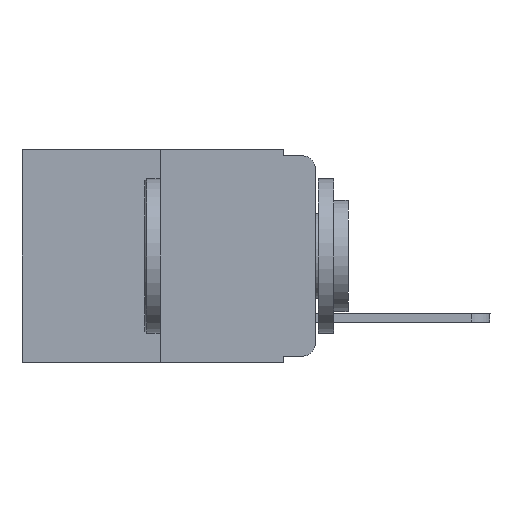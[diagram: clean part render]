
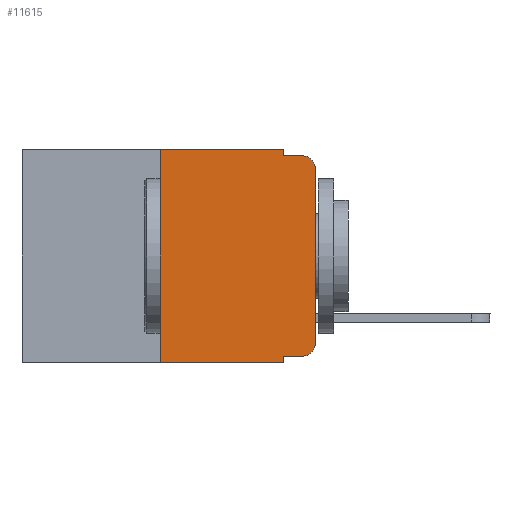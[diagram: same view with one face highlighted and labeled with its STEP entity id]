
A CAD part, left-side view. The second image highlights one B-rep face of the part: STEP entity #11615.
In plain terms, the highlighted planar face has unit normal (-1, 0, 0).
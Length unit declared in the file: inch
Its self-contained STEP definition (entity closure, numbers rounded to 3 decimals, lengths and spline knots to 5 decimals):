
#51 = DIRECTION ( 'NONE',  ( 0., 0., -1. ) ) ;
#181 = CARTESIAN_POINT ( 'NONE',  ( 0., 0.25, 0. ) ) ;
#511 = ORIENTED_EDGE ( 'NONE', *, *, #19440, .T. ) ;
#633 = VECTOR ( 'NONE', #51, 39.37008 ) ;
#698 = VERTEX_POINT ( 'NONE', #17867 ) ;
#1105 = VECTOR ( 'NONE', #6420, 39.37008 ) ;
#1131 = DIRECTION ( 'NONE',  ( 0., 0., -1. ) ) ;
#1224 = VERTEX_POINT ( 'NONE', #16883 ) ;
#1308 = VERTEX_POINT ( 'NONE', #9036 ) ;
#1438 = ORIENTED_EDGE ( 'NONE', *, *, #10637, .F. ) ;
#1750 = DIRECTION ( 'NONE',  ( 0., 0., 1. ) ) ;
#1753 = CARTESIAN_POINT ( 'NONE',  ( 0., 0., 0. ) ) ;
#1965 = EDGE_CURVE ( 'NONE', #13416, #4451, #17871, .T. ) ;
#2322 = CARTESIAN_POINT ( 'NONE',  ( 0., 0.473, -0.343 ) ) ;
#3018 = EDGE_CURVE ( 'NONE', #4451, #4142, #10942, .T. ) ;
#3099 = CARTESIAN_POINT ( 'NONE',  ( 0., 0., -0.313 ) ) ;
#4028 = VERTEX_POINT ( 'NONE', #3099 ) ;
#4041 = CARTESIAN_POINT ( 'NONE',  ( 0., 0.051, -0.01 ) ) ;
#4138 = LINE ( 'NONE', #4041, #8868 ) ;
#4142 = VERTEX_POINT ( 'NONE', #10747 ) ;
#4255 = VECTOR ( 'NONE', #10117, 39.37008 ) ;
#4418 = LINE ( 'NONE', #1753, #1105 ) ;
#4450 = EDGE_CURVE ( 'NONE', #16746, #13416, #20110, .T. ) ;
#4451 = VERTEX_POINT ( 'NONE', #11332 ) ;
#4659 = CARTESIAN_POINT ( 'NONE',  ( 0., 0.051, 0. ) ) ;
#5039 = DIRECTION ( 'NONE',  ( 0., 0., -1. ) ) ;
#5321 = VECTOR ( 'NONE', #13390, 39.37008 ) ;
#5328 = ORIENTED_EDGE ( 'NONE', *, *, #3018, .F. ) ;
#5369 = DIRECTION ( 'NONE',  ( -1., 0., 0. ) ) ;
#5661 = ORIENTED_EDGE ( 'NONE', *, *, #4450, .F. ) ;
#5668 = VECTOR ( 'NONE', #8536, 39.37008 ) ;
#5938 = CIRCLE ( 'NONE', #19613, 0.02 ) ;
#5996 = CARTESIAN_POINT ( 'NONE',  ( 0., 0.25, -0.343 ) ) ;
#6420 = DIRECTION ( 'NONE',  ( 0., 0., 1. ) ) ;
#6889 = EDGE_CURVE ( 'NONE', #12140, #4028, #10310, .T. ) ;
#8536 = DIRECTION ( 'NONE',  ( 0., -1., 0. ) ) ;
#8677 = PLANE ( 'NONE',  #17695 ) ;
#8794 = ORIENTED_EDGE ( 'NONE', *, *, #6889, .T. ) ;
#8868 = VECTOR ( 'NONE', #10045, 39.37008 ) ;
#9036 = CARTESIAN_POINT ( 'NONE',  ( 0., 0.051, -0.343 ) ) ;
#9367 = ORIENTED_EDGE ( 'NONE', *, *, #1965, .F. ) ;
#9650 = EDGE_CURVE ( 'NONE', #1224, #698, #5938, .T. ) ;
#9795 = ORIENTED_EDGE ( 'NONE', *, *, #11631, .T. ) ;
#10045 = DIRECTION ( 'NONE',  ( 0., -1., 0. ) ) ;
#10117 = DIRECTION ( 'NONE',  ( 0., -1., 0. ) ) ;
#10310 = CIRCLE ( 'NONE', #14862, 0.02 ) ;
#10389 = ORIENTED_EDGE ( 'NONE', *, *, #20012, .T. ) ;
#10637 = EDGE_CURVE ( 'NONE', #4142, #698, #4138, .T. ) ;
#10747 = CARTESIAN_POINT ( 'NONE',  ( 0., 0.051, -0.01 ) ) ;
#10942 = LINE ( 'NONE', #14113, #16227 ) ;
#11332 = CARTESIAN_POINT ( 'NONE',  ( 0., 0.051, 0. ) ) ;
#11613 = LINE ( 'NONE', #2322, #5668 ) ;
#11615 = ADVANCED_FACE ( 'NONE', ( #18163 ), #8677, .F. ) ;
#11631 = EDGE_CURVE ( 'NONE', #19550, #12140, #19896, .T. ) ;
#12140 = VERTEX_POINT ( 'NONE', #12539 ) ;
#12160 = CARTESIAN_POINT ( 'NONE',  ( 0., 0.473, 0. ) ) ;
#12397 = DIRECTION ( 'NONE',  ( -1., 0., 0. ) ) ;
#12499 = DIRECTION ( 'NONE',  ( 0., 0., -1. ) ) ;
#12539 = CARTESIAN_POINT ( 'NONE',  ( 0., 0.02, -0.333 ) ) ;
#13133 = DIRECTION ( 'NONE',  ( 0., 0., -1. ) ) ;
#13390 = DIRECTION ( 'NONE',  ( 0., -1., 0. ) ) ;
#13416 = VERTEX_POINT ( 'NONE', #181 ) ;
#13949 = EDGE_CURVE ( 'NONE', #19550, #1308, #18615, .T. ) ;
#14113 = CARTESIAN_POINT ( 'NONE',  ( 0., 0.051, 0. ) ) ;
#14719 = ORIENTED_EDGE ( 'NONE', *, *, #9650, .T. ) ;
#14862 = AXIS2_PLACEMENT_3D ( 'NONE', #16086, #5369, #13133 ) ;
#15304 = ORIENTED_EDGE ( 'NONE', *, *, #13949, .F. ) ;
#15917 = VECTOR ( 'NONE', #1750, 39.37008 ) ;
#16086 = CARTESIAN_POINT ( 'NONE',  ( 0., 0.02, -0.313 ) ) ;
#16227 = VECTOR ( 'NONE', #5039, 39.37008 ) ;
#16423 = EDGE_LOOP ( 'NONE', ( #10389, #14719, #1438, #5328, #9367, #5661, #511, #15304, #9795, #8794 ) ) ;
#16591 = CARTESIAN_POINT ( 'NONE',  ( 0., 0.051, -0.333 ) ) ;
#16628 = DIRECTION ( 'NONE',  ( 1., 0., 0. ) ) ;
#16746 = VERTEX_POINT ( 'NONE', #5996 ) ;
#16883 = CARTESIAN_POINT ( 'NONE',  ( 0., 0., -0.03 ) ) ;
#17235 = CARTESIAN_POINT ( 'NONE',  ( 0., 0.25, 0. ) ) ;
#17695 = AXIS2_PLACEMENT_3D ( 'NONE', #12160, #16628, #1131 ) ;
#17867 = CARTESIAN_POINT ( 'NONE',  ( 0., 0.02, -0.01 ) ) ;
#17871 = LINE ( 'NONE', #19208, #4255 ) ;
#18070 = CARTESIAN_POINT ( 'NONE',  ( 0., 0.051, -0.333 ) ) ;
#18163 = FACE_OUTER_BOUND ( 'NONE', #16423, .T. ) ;
#18595 = CARTESIAN_POINT ( 'NONE',  ( 0., 0.02, -0.03 ) ) ;
#18615 = LINE ( 'NONE', #4659, #633 ) ;
#19208 = CARTESIAN_POINT ( 'NONE',  ( 0., 0.473, 0. ) ) ;
#19440 = EDGE_CURVE ( 'NONE', #16746, #1308, #11613, .T. ) ;
#19550 = VERTEX_POINT ( 'NONE', #16591 ) ;
#19613 = AXIS2_PLACEMENT_3D ( 'NONE', #18595, #12397, #12499 ) ;
#19896 = LINE ( 'NONE', #18070, #5321 ) ;
#20012 = EDGE_CURVE ( 'NONE', #4028, #1224, #4418, .T. ) ;
#20110 = LINE ( 'NONE', #17235, #15917 ) ;
